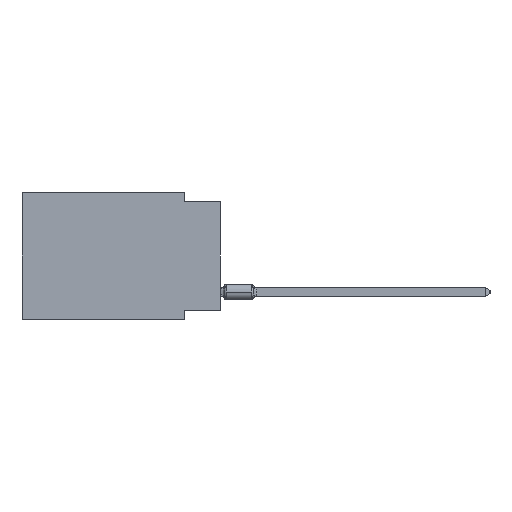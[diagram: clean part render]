
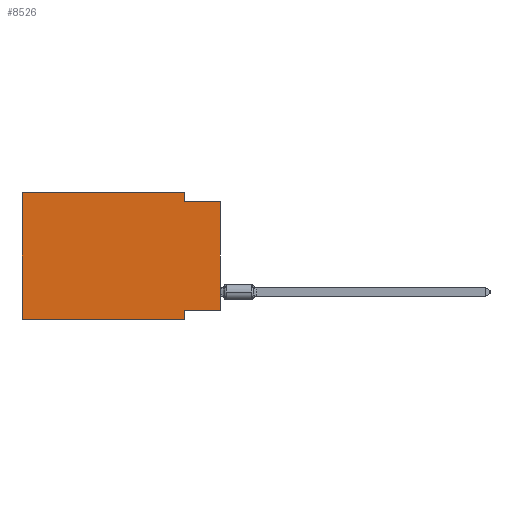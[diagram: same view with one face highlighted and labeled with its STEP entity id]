
A CAD part, left-side view. The second image highlights one B-rep face of the part: STEP entity #8526.
In plain terms, the highlighted planar face has unit normal (-1, 0, 0).
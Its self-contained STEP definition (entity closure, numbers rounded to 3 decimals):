
#80 = CARTESIAN_POINT ( 'NONE',  ( 0., 2.54, 0. ) ) ;
#146 = EDGE_LOOP ( 'NONE', ( #20291, #14185, #20358, #3928, #18986, #2687, #20086, #10653 ) ) ;
#690 = VECTOR ( 'NONE', #7685, 1000. ) ;
#1643 = CARTESIAN_POINT ( 'NONE',  ( 0., 0., -0.635 ) ) ;
#2279 = CARTESIAN_POINT ( 'NONE',  ( 0., 13.97, 0. ) ) ;
#2386 = DIRECTION ( 'NONE',  ( 0., 0., 1. ) ) ;
#2550 = PLANE ( 'NONE',  #12828 ) ;
#2687 = ORIENTED_EDGE ( 'NONE', *, *, #20333, .T. ) ;
#3106 = VERTEX_POINT ( 'NONE', #15461 ) ;
#3818 = VERTEX_POINT ( 'NONE', #6264 ) ;
#3928 = ORIENTED_EDGE ( 'NONE', *, *, #4305, .F. ) ;
#4115 = VECTOR ( 'NONE', #6591, 1000. ) ;
#4305 = EDGE_CURVE ( 'NONE', #5074, #10992, #13108, .T. ) ;
#4942 = DIRECTION ( 'NONE',  ( 0., 0., 1. ) ) ;
#5074 = VERTEX_POINT ( 'NONE', #16150 ) ;
#5138 = VERTEX_POINT ( 'NONE', #10652 ) ;
#5666 = DIRECTION ( 'NONE',  ( 0., 1., 0. ) ) ;
#6097 = EDGE_CURVE ( 'NONE', #3106, #3818, #10496, .T. ) ;
#6264 = CARTESIAN_POINT ( 'NONE',  ( 0., 2.54, -8.255 ) ) ;
#6315 = DIRECTION ( 'NONE',  ( 0., 0., -1. ) ) ;
#6532 = VECTOR ( 'NONE', #8389, 1000. ) ;
#6591 = DIRECTION ( 'NONE',  ( 0., 0., -1. ) ) ;
#7465 = DIRECTION ( 'NONE',  ( 0., 0., -1. ) ) ;
#7685 = DIRECTION ( 'NONE',  ( 0., -1., 0. ) ) ;
#8103 = LINE ( 'NONE', #14432, #16426 ) ;
#8389 = DIRECTION ( 'NONE',  ( 0., -1., 0. ) ) ;
#8526 = ADVANCED_FACE ( 'NONE', ( #17252 ), #2550, .F. ) ;
#9075 = CARTESIAN_POINT ( 'NONE',  ( 0., 13.97, 0. ) ) ;
#9390 = LINE ( 'NONE', #9689, #690 ) ;
#9536 = EDGE_CURVE ( 'NONE', #3106, #19553, #16219, .T. ) ;
#9689 = CARTESIAN_POINT ( 'NONE',  ( 0., 13.97, -8.89 ) ) ;
#10496 = LINE ( 'NONE', #16728, #12755 ) ;
#10652 = CARTESIAN_POINT ( 'NONE',  ( 0., 2.54, -8.89 ) ) ;
#10653 = ORIENTED_EDGE ( 'NONE', *, *, #6097, .F. ) ;
#10781 = DIRECTION ( 'NONE',  ( 1., 0., 0. ) ) ;
#10825 = LINE ( 'NONE', #2279, #20338 ) ;
#10833 = VERTEX_POINT ( 'NONE', #20591 ) ;
#10992 = VERTEX_POINT ( 'NONE', #10996 ) ;
#10996 = CARTESIAN_POINT ( 'NONE',  ( 0., 2.54, 0. ) ) ;
#11151 = LINE ( 'NONE', #12658, #12856 ) ;
#12658 = CARTESIAN_POINT ( 'NONE',  ( 0., 2.54, -8.89 ) ) ;
#12755 = VECTOR ( 'NONE', #5666, 1000. ) ;
#12828 = AXIS2_PLACEMENT_3D ( 'NONE', #9075, #10781, #7465 ) ;
#12856 = VECTOR ( 'NONE', #6315, 1000. ) ;
#12978 = CARTESIAN_POINT ( 'NONE',  ( 0., 0., 0. ) ) ;
#13108 = LINE ( 'NONE', #17976, #6532 ) ;
#14185 = ORIENTED_EDGE ( 'NONE', *, *, #20290, .F. ) ;
#14412 = VERTEX_POINT ( 'NONE', #16588 ) ;
#14432 = CARTESIAN_POINT ( 'NONE',  ( 0., 0., -0.635 ) ) ;
#14760 = LINE ( 'NONE', #80, #4115 ) ;
#15461 = CARTESIAN_POINT ( 'NONE',  ( 0., 0., -8.255 ) ) ;
#16028 = EDGE_CURVE ( 'NONE', #14412, #5074, #10825, .T. ) ;
#16150 = CARTESIAN_POINT ( 'NONE',  ( 0., 13.97, 0. ) ) ;
#16219 = LINE ( 'NONE', #12978, #21064 ) ;
#16426 = VECTOR ( 'NONE', #20748, 1000. ) ;
#16588 = CARTESIAN_POINT ( 'NONE',  ( 0., 13.97, -8.89 ) ) ;
#16728 = CARTESIAN_POINT ( 'NONE',  ( 0., 0., -8.255 ) ) ;
#17252 = FACE_OUTER_BOUND ( 'NONE', #146, .T. ) ;
#17778 = EDGE_CURVE ( 'NONE', #3818, #5138, #11151, .T. ) ;
#17976 = CARTESIAN_POINT ( 'NONE',  ( 0., 13.97, 0. ) ) ;
#18986 = ORIENTED_EDGE ( 'NONE', *, *, #16028, .F. ) ;
#19553 = VERTEX_POINT ( 'NONE', #1643 ) ;
#20086 = ORIENTED_EDGE ( 'NONE', *, *, #17778, .F. ) ;
#20290 = EDGE_CURVE ( 'NONE', #10833, #19553, #8103, .T. ) ;
#20291 = ORIENTED_EDGE ( 'NONE', *, *, #9536, .T. ) ;
#20333 = EDGE_CURVE ( 'NONE', #14412, #5138, #9390, .T. ) ;
#20338 = VECTOR ( 'NONE', #2386, 1000. ) ;
#20358 = ORIENTED_EDGE ( 'NONE', *, *, #20368, .F. ) ;
#20368 = EDGE_CURVE ( 'NONE', #10992, #10833, #14760, .T. ) ;
#20591 = CARTESIAN_POINT ( 'NONE',  ( 0., 2.54, -0.635 ) ) ;
#20748 = DIRECTION ( 'NONE',  ( 0., -1., 0. ) ) ;
#21064 = VECTOR ( 'NONE', #4942, 1000. ) ;
